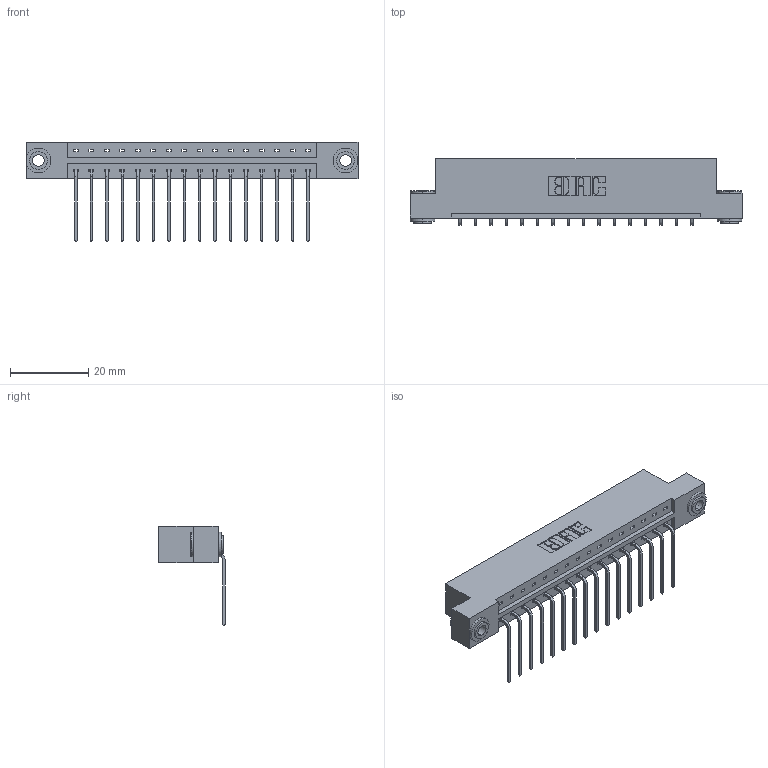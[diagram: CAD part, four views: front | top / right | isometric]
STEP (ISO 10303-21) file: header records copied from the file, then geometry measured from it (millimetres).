
FILE_DESCRIPTION (( 'STEP AP203' ), '1' );
FILE_NAME ('833-016-559-103.STEP', '2020-05-31T19:05:36', ( '' ), ( '' ), 'SwSTEP 2.0', 'SolidWorks 2020', '' );
FILE_SCHEMA (( 'CONFIG_CONTROL_DESIGN' ));
Length unit declared in the file: inch
Products named in the file (4): 345-250-002_345-250-002-102; 345-292-001_558 559 Tail - 1; 833 Part_Flush - .156 Dia - TH; 833-016-559-103
Assembly tree (19 placements, depth 2):
  833-016-559-103
    833 Part_Flush - .156 Dia - TH
    345-292-001_558 559 Tail - 1  x16
    345-250-002_345-250-002-102  x2
Bounding box: 84.94 x 17.09 x 25.53 mm (x, y, z)
Volume: 8396.2 mm3; surface area: 9468.8 mm2
Topology: 19 solids, 19 shells, 1112 faces, 3299 edges, 2174 vertices
Faces by surface type: plane 784, cylinder 320, cone 8
Entity records: 13878 total; most frequent: CARTESIAN_POINT 2377, ORIENTED_EDGE 2322, DIRECTION 2091, EDGE_CURVE 1161, LINE 1009, VECTOR 1009, VERTEX_POINT 770, AXIS2_PLACEMENT_3D 541
